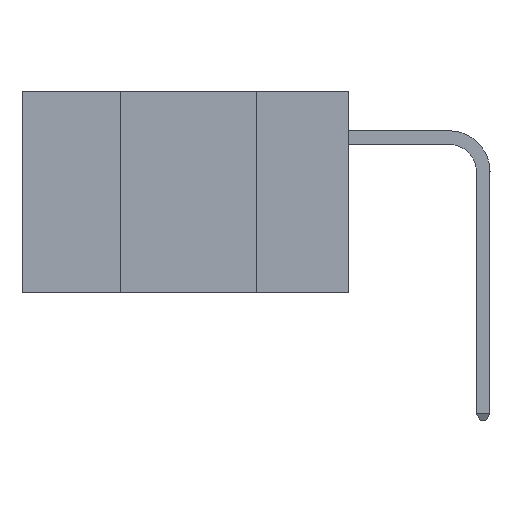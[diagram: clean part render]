
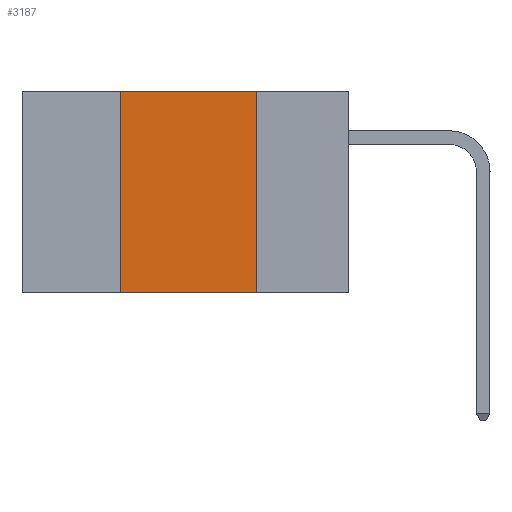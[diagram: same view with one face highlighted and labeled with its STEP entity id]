
A CAD part, left-side view. The second image highlights one B-rep face of the part: STEP entity #3187.
In plain terms, the highlighted planar face has unit normal (-1, 0, 0).
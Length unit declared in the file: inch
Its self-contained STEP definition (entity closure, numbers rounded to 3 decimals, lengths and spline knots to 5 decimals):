
#173 = VECTOR ( 'NONE', #2089, 39.37008 ) ;
#1307 = LINE ( 'NONE', #12165, #9913 ) ;
#1894 = DIRECTION ( 'NONE',  ( 0., 0., -1. ) ) ;
#2089 = DIRECTION ( 'NONE',  ( 0., -1., 0. ) ) ;
#2921 = CARTESIAN_POINT ( 'NONE',  ( 0., 0.6, 0. ) ) ;
#2925 = VECTOR ( 'NONE', #21174, 39.37008 ) ;
#3187 = ADVANCED_FACE ( 'NONE', ( #16965 ), #8889, .F. ) ;
#3697 = VERTEX_POINT ( 'NONE', #3995 ) ;
#3758 = EDGE_CURVE ( 'NONE', #3697, #13486, #13859, .T. ) ;
#3995 = CARTESIAN_POINT ( 'NONE',  ( 0., 0.42, 0. ) ) ;
#5089 = EDGE_CURVE ( 'NONE', #19354, #3697, #16105, .T. ) ;
#6138 = CARTESIAN_POINT ( 'NONE',  ( 0., 0.6, 0. ) ) ;
#7357 = CARTESIAN_POINT ( 'NONE',  ( 0., 0.42, -0.37 ) ) ;
#8444 = EDGE_CURVE ( 'NONE', #13486, #16826, #1307, .T. ) ;
#8768 = DIRECTION ( 'NONE',  ( 0., 0., -1. ) ) ;
#8828 = ORIENTED_EDGE ( 'NONE', *, *, #3758, .F. ) ;
#8889 = PLANE ( 'NONE',  #18247 ) ;
#9416 = CARTESIAN_POINT ( 'NONE',  ( 0., 0.6, -0.37 ) ) ;
#9896 = ORIENTED_EDGE ( 'NONE', *, *, #8444, .F. ) ;
#9913 = VECTOR ( 'NONE', #8768, 39.37008 ) ;
#10728 = EDGE_CURVE ( 'NONE', #19354, #16826, #20797, .T. ) ;
#11684 = VECTOR ( 'NONE', #18732, 39.37008 ) ;
#12165 = CARTESIAN_POINT ( 'NONE',  ( 0., 0.17, 0. ) ) ;
#12306 = CARTESIAN_POINT ( 'NONE',  ( 0., 0.17, -0.37 ) ) ;
#13486 = VERTEX_POINT ( 'NONE', #19985 ) ;
#13859 = LINE ( 'NONE', #2921, #173 ) ;
#15866 = DIRECTION ( 'NONE',  ( 1., 0., 0. ) ) ;
#16105 = LINE ( 'NONE', #20997, #11684 ) ;
#16826 = VERTEX_POINT ( 'NONE', #12306 ) ;
#16965 = FACE_OUTER_BOUND ( 'NONE', #20692, .T. ) ;
#17721 = ORIENTED_EDGE ( 'NONE', *, *, #5089, .F. ) ;
#18247 = AXIS2_PLACEMENT_3D ( 'NONE', #6138, #15866, #1894 ) ;
#18732 = DIRECTION ( 'NONE',  ( 0., 0., 1. ) ) ;
#19354 = VERTEX_POINT ( 'NONE', #7357 ) ;
#19985 = CARTESIAN_POINT ( 'NONE',  ( 0., 0.17, 0. ) ) ;
#20692 = EDGE_LOOP ( 'NONE', ( #9896, #8828, #17721, #21713 ) ) ;
#20797 = LINE ( 'NONE', #9416, #2925 ) ;
#20997 = CARTESIAN_POINT ( 'NONE',  ( 0., 0.42, 0. ) ) ;
#21174 = DIRECTION ( 'NONE',  ( 0., -1., 0. ) ) ;
#21713 = ORIENTED_EDGE ( 'NONE', *, *, #10728, .T. ) ;
